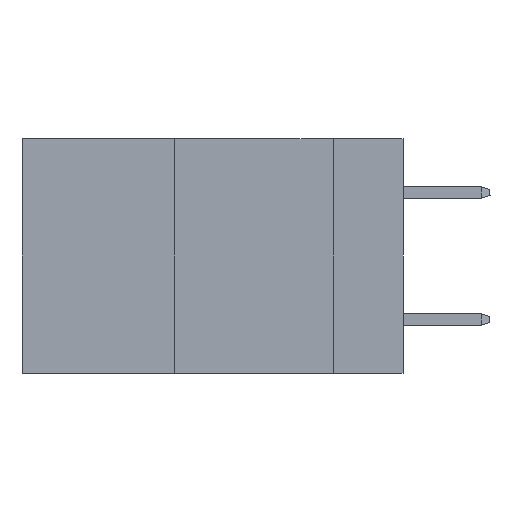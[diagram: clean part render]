
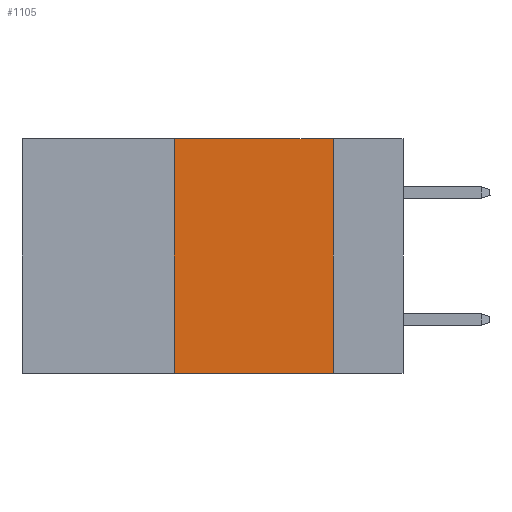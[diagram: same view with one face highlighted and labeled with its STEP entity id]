
A CAD part, left-side view. The second image highlights one B-rep face of the part: STEP entity #1105.
In plain terms, the highlighted planar face has unit normal (-1, 0, 0).
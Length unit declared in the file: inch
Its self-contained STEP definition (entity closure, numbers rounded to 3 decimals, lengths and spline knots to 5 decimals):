
#585 = VECTOR ( 'NONE', #42747, 39.37008 ) ;
#1105 = ADVANCED_FACE ( 'NONE', ( #12357 ), #29573, .F. ) ;
#1306 = CARTESIAN_POINT ( 'NONE',  ( 0., 0.11, 0. ) ) ;
#2444 = EDGE_LOOP ( 'NONE', ( #18653, #27519, #20830, #22870 ) ) ;
#5392 = CARTESIAN_POINT ( 'NONE',  ( 0., 0.36, 0. ) ) ;
#9373 = VERTEX_POINT ( 'NONE', #1306 ) ;
#10450 = CARTESIAN_POINT ( 'NONE',  ( 0., 0.11, -0.37 ) ) ;
#11138 = VERTEX_POINT ( 'NONE', #21684 ) ;
#12302 = CARTESIAN_POINT ( 'NONE',  ( 0., 0.6, -0.37 ) ) ;
#12357 = FACE_OUTER_BOUND ( 'NONE', #2444, .T. ) ;
#18007 = VECTOR ( 'NONE', #41436, 39.37008 ) ;
#18285 = VERTEX_POINT ( 'NONE', #10450 ) ;
#18653 = ORIENTED_EDGE ( 'NONE', *, *, #35266, .F. ) ;
#20830 = ORIENTED_EDGE ( 'NONE', *, *, #24592, .F. ) ;
#21684 = CARTESIAN_POINT ( 'NONE',  ( 0., 0.36, -0.37 ) ) ;
#21766 = DIRECTION ( 'NONE',  ( 0., 0., -1. ) ) ;
#22870 = ORIENTED_EDGE ( 'NONE', *, *, #25031, .T. ) ;
#24592 = EDGE_CURVE ( 'NONE', #11138, #30244, #43025, .T. ) ;
#25031 = EDGE_CURVE ( 'NONE', #11138, #18285, #25733, .T. ) ;
#25124 = DIRECTION ( 'NONE',  ( 1., 0., 0. ) ) ;
#25637 = VECTOR ( 'NONE', #42589, 39.37008 ) ;
#25733 = LINE ( 'NONE', #12302, #585 ) ;
#27391 = CARTESIAN_POINT ( 'NONE',  ( 0., 0.36, 0. ) ) ;
#27519 = ORIENTED_EDGE ( 'NONE', *, *, #40619, .F. ) ;
#28501 = AXIS2_PLACEMENT_3D ( 'NONE', #32964, #25124, #21766 ) ;
#29573 = PLANE ( 'NONE',  #28501 ) ;
#30244 = VERTEX_POINT ( 'NONE', #27391 ) ;
#30963 = LINE ( 'NONE', #34114, #37177 ) ;
#31143 = CARTESIAN_POINT ( 'NONE',  ( 0., 0.6, 0. ) ) ;
#32964 = CARTESIAN_POINT ( 'NONE',  ( 0., 0.6, 0. ) ) ;
#33904 = DIRECTION ( 'NONE',  ( 0., 0., -1. ) ) ;
#34114 = CARTESIAN_POINT ( 'NONE',  ( 0., 0.11, 0. ) ) ;
#35266 = EDGE_CURVE ( 'NONE', #9373, #18285, #30963, .T. ) ;
#37177 = VECTOR ( 'NONE', #33904, 39.37008 ) ;
#38786 = LINE ( 'NONE', #31143, #18007 ) ;
#40619 = EDGE_CURVE ( 'NONE', #30244, #9373, #38786, .T. ) ;
#41436 = DIRECTION ( 'NONE',  ( 0., -1., 0. ) ) ;
#42589 = DIRECTION ( 'NONE',  ( 0., 0., 1. ) ) ;
#42747 = DIRECTION ( 'NONE',  ( 0., -1., 0. ) ) ;
#43025 = LINE ( 'NONE', #5392, #25637 ) ;
